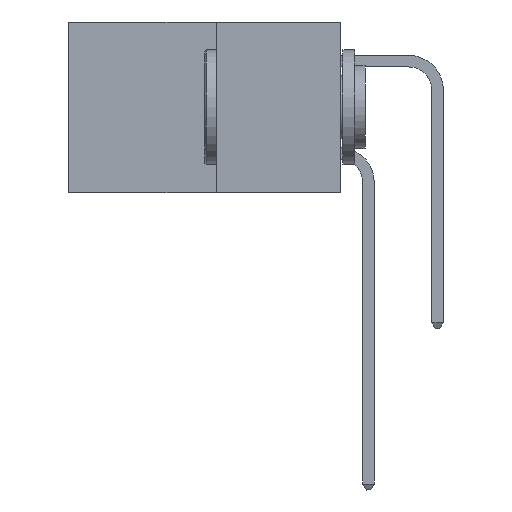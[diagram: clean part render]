
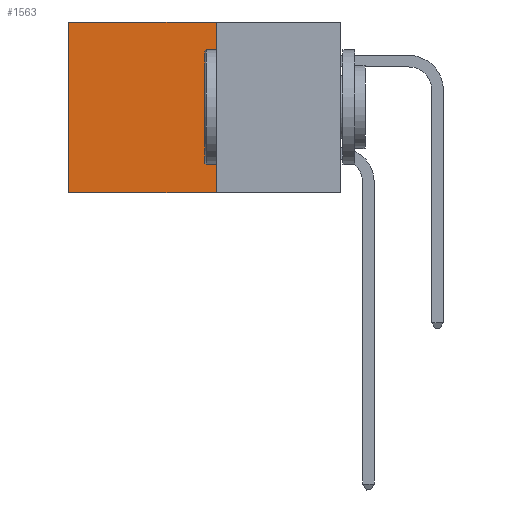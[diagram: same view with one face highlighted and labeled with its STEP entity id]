
A CAD part, left-side view. The second image highlights one B-rep face of the part: STEP entity #1563.
In plain terms, the highlighted planar face has unit normal (-1, 0, 0).
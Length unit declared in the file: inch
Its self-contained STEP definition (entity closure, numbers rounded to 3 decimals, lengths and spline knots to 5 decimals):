
#565 = VECTOR ( 'NONE', #12848, 39.37008 ) ;
#1067 = FACE_OUTER_BOUND ( 'NONE', #3910, .T. ) ;
#1228 = LINE ( 'NONE', #22951, #565 ) ;
#1563 = ADVANCED_FACE ( 'NONE', ( #1067 ), #23090, .F. ) ;
#3910 = EDGE_LOOP ( 'NONE', ( #25979, #22383, #20641, #24521 ) ) ;
#5427 = VECTOR ( 'NONE', #24380, 39.37008 ) ;
#7028 = VERTEX_POINT ( 'NONE', #13119 ) ;
#9615 = CARTESIAN_POINT ( 'NONE',  ( 0.277, 0.27, 0. ) ) ;
#10269 = CARTESIAN_POINT ( 'NONE',  ( 0.277, 0.27, -0.37 ) ) ;
#10417 = CARTESIAN_POINT ( 'NONE',  ( 0.277, 0.59, -0.37 ) ) ;
#10506 = CARTESIAN_POINT ( 'NONE',  ( 0.277, 0.59, -0.37 ) ) ;
#11054 = VECTOR ( 'NONE', #11683, 39.37008 ) ;
#11675 = LINE ( 'NONE', #9615, #11054 ) ;
#11683 = DIRECTION ( 'NONE',  ( 0., 1., 0. ) ) ;
#12459 = DIRECTION ( 'NONE',  ( 0., 0., -1. ) ) ;
#12848 = DIRECTION ( 'NONE',  ( 0., 0., -1. ) ) ;
#13119 = CARTESIAN_POINT ( 'NONE',  ( 0.277, 0.59, 0. ) ) ;
#15338 = CARTESIAN_POINT ( 'NONE',  ( 0.277, 0.27, -0.37 ) ) ;
#15470 = VECTOR ( 'NONE', #12459, 39.37008 ) ;
#16098 = LINE ( 'NONE', #10417, #15470 ) ;
#16352 = EDGE_CURVE ( 'NONE', #24595, #17898, #1228, .T. ) ;
#16382 = CARTESIAN_POINT ( 'NONE',  ( 0.277, 0.27, -0.37 ) ) ;
#16892 = LINE ( 'NONE', #10269, #5427 ) ;
#17898 = VERTEX_POINT ( 'NONE', #16382 ) ;
#19496 = CARTESIAN_POINT ( 'NONE',  ( 0.277, 0.27, 0. ) ) ;
#19800 = EDGE_CURVE ( 'NONE', #17898, #22940, #16892, .T. ) ;
#20641 = ORIENTED_EDGE ( 'NONE', *, *, #16352, .F. ) ;
#20704 = AXIS2_PLACEMENT_3D ( 'NONE', #15338, #26159, #20741 ) ;
#20741 = DIRECTION ( 'NONE',  ( 0., 0., -1. ) ) ;
#22383 = ORIENTED_EDGE ( 'NONE', *, *, #19800, .F. ) ;
#22664 = EDGE_CURVE ( 'NONE', #24595, #7028, #11675, .T. ) ;
#22909 = EDGE_CURVE ( 'NONE', #7028, #22940, #16098, .T. ) ;
#22940 = VERTEX_POINT ( 'NONE', #10506 ) ;
#22951 = CARTESIAN_POINT ( 'NONE',  ( 0.277, 0.27, -0.37 ) ) ;
#23090 = PLANE ( 'NONE',  #20704 ) ;
#24380 = DIRECTION ( 'NONE',  ( 0., 1., 0. ) ) ;
#24521 = ORIENTED_EDGE ( 'NONE', *, *, #22664, .T. ) ;
#24595 = VERTEX_POINT ( 'NONE', #19496 ) ;
#25979 = ORIENTED_EDGE ( 'NONE', *, *, #22909, .T. ) ;
#26159 = DIRECTION ( 'NONE',  ( 1., 0., 0. ) ) ;
